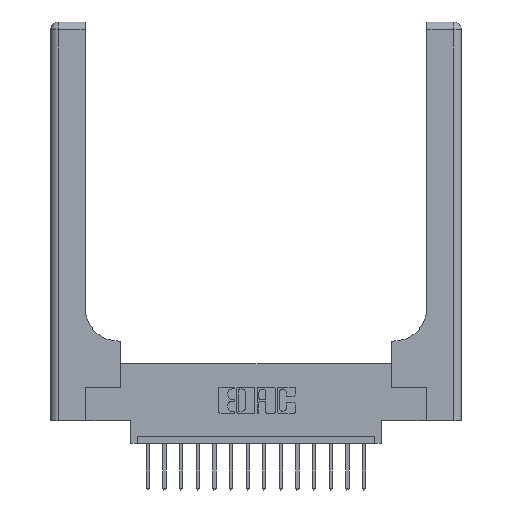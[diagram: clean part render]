
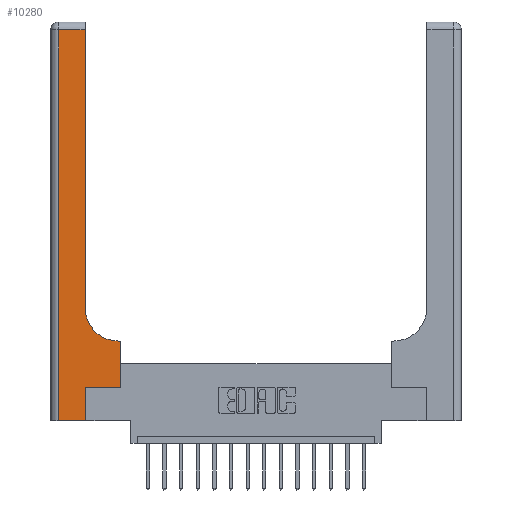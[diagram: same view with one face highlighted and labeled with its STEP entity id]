
A CAD part, top view. The second image highlights one B-rep face of the part: STEP entity #10280.
In plain terms, the highlighted planar face has unit normal (0, 0, 1).
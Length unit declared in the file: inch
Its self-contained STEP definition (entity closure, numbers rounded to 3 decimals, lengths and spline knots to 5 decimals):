
#17 = VERTEX_POINT ( 'NONE', #7320 ) ;
#414 = ORIENTED_EDGE ( 'NONE', *, *, #18149, .T. ) ;
#710 = VERTEX_POINT ( 'NONE', #17041 ) ;
#808 = EDGE_CURVE ( 'NONE', #9698, #7693, #7639, .T. ) ;
#989 = CARTESIAN_POINT ( 'NONE',  ( 0.06, 3., 0.37 ) ) ;
#1818 = ORIENTED_EDGE ( 'NONE', *, *, #17725, .T. ) ;
#1839 = CARTESIAN_POINT ( 'NONE',  ( 0., 3., 0.37 ) ) ;
#2275 = EDGE_CURVE ( 'NONE', #710, #17, #11465, .T. ) ;
#2359 = DIRECTION ( 'NONE',  ( 1., 0., 0. ) ) ;
#2383 = ORIENTED_EDGE ( 'NONE', *, *, #7016, .T. ) ;
#2452 = EDGE_CURVE ( 'NONE', #14809, #3536, #15968, .T. ) ;
#2605 = DIRECTION ( 'NONE',  ( 0., 0., -1. ) ) ;
#2976 = DIRECTION ( 'NONE',  ( 0., 1., 0. ) ) ;
#3241 = CARTESIAN_POINT ( 'NONE',  ( 0.265, 0., 0.37 ) ) ;
#3349 = DIRECTION ( 'NONE',  ( -1., 0., 0. ) ) ;
#3536 = VERTEX_POINT ( 'NONE', #13038 ) ;
#3635 = VERTEX_POINT ( 'NONE', #6782 ) ;
#3648 = CARTESIAN_POINT ( 'NONE',  ( 0.265, 0.25, 0.37 ) ) ;
#3989 = FACE_OUTER_BOUND ( 'NONE', #7374, .T. ) ;
#4073 = VERTEX_POINT ( 'NONE', #6824 ) ;
#4450 = ORIENTED_EDGE ( 'NONE', *, *, #2275, .T. ) ;
#4455 = ORIENTED_EDGE ( 'NONE', *, *, #808, .T. ) ;
#4923 = DIRECTION ( 'NONE',  ( -1., 0., 0. ) ) ;
#5470 = DIRECTION ( 'NONE',  ( -1., 0., 0. ) ) ;
#6045 = VECTOR ( 'NONE', #2976, 39.37008 ) ;
#6355 = CARTESIAN_POINT ( 'NONE',  ( 0.528, 0.25, 0.37 ) ) ;
#6574 = LINE ( 'NONE', #13385, #10532 ) ;
#6782 = CARTESIAN_POINT ( 'NONE',  ( 0.265, 0.25, 0.37 ) ) ;
#6824 = CARTESIAN_POINT ( 'NONE',  ( 0.528, 0.25, 0.37 ) ) ;
#7016 = EDGE_CURVE ( 'NONE', #3536, #710, #18098, .T. ) ;
#7320 = CARTESIAN_POINT ( 'NONE',  ( 0.26, 2.94, 0.37 ) ) ;
#7374 = EDGE_LOOP ( 'NONE', ( #4450, #15392, #4455, #16067, #1818, #414, #14215, #13484, #2383 ) ) ;
#7639 = LINE ( 'NONE', #989, #13537 ) ;
#7693 = VERTEX_POINT ( 'NONE', #14529 ) ;
#7717 = LINE ( 'NONE', #6355, #16822 ) ;
#7744 = EDGE_CURVE ( 'NONE', #4073, #14809, #7717, .T. ) ;
#8080 = CARTESIAN_POINT ( 'NONE',  ( 0.528, 0.6, 0.37 ) ) ;
#8204 = CARTESIAN_POINT ( 'NONE',  ( 0.265, 0., 0.37 ) ) ;
#8979 = CARTESIAN_POINT ( 'NONE',  ( 0.26, 0.6, 0.37 ) ) ;
#9279 = DIRECTION ( 'NONE',  ( 1., 0., 0. ) ) ;
#9527 = AXIS2_PLACEMENT_3D ( 'NONE', #1839, #2605, #5470 ) ;
#9698 = VERTEX_POINT ( 'NONE', #17572 ) ;
#9958 = VECTOR ( 'NONE', #13180, 39.37008 ) ;
#10175 = AXIS2_PLACEMENT_3D ( 'NONE', #11846, #11935, #9279 ) ;
#10280 = ADVANCED_FACE ( 'NONE', ( #3989 ), #12453, .F. ) ;
#10532 = VECTOR ( 'NONE', #4923, 39.37008 ) ;
#11465 = LINE ( 'NONE', #12646, #6045 ) ;
#11846 = CARTESIAN_POINT ( 'NONE',  ( 0.51, 0.85, 0.37 ) ) ;
#11883 = VERTEX_POINT ( 'NONE', #8204 ) ;
#11935 = DIRECTION ( 'NONE',  ( 0., 0., -1. ) ) ;
#12453 = PLANE ( 'NONE',  #9527 ) ;
#12646 = CARTESIAN_POINT ( 'NONE',  ( 0.26, 3., 0.37 ) ) ;
#13038 = CARTESIAN_POINT ( 'NONE',  ( 0.51, 0.6, 0.37 ) ) ;
#13091 = VECTOR ( 'NONE', #3349, 39.37008 ) ;
#13180 = DIRECTION ( 'NONE',  ( 0., 1., 0. ) ) ;
#13204 = VECTOR ( 'NONE', #2359, 39.37008 ) ;
#13230 = LINE ( 'NONE', #3648, #13204 ) ;
#13385 = CARTESIAN_POINT ( 'NONE',  ( 0., 2.94, 0.37 ) ) ;
#13432 = DIRECTION ( 'NONE',  ( 0., 1., 0. ) ) ;
#13484 = ORIENTED_EDGE ( 'NONE', *, *, #2452, .T. ) ;
#13537 = VECTOR ( 'NONE', #14901, 39.37008 ) ;
#14215 = ORIENTED_EDGE ( 'NONE', *, *, #7744, .T. ) ;
#14509 = DIRECTION ( 'NONE',  ( 1., 0., 0. ) ) ;
#14529 = CARTESIAN_POINT ( 'NONE',  ( 0.06, 0., 0.37 ) ) ;
#14809 = VERTEX_POINT ( 'NONE', #8080 ) ;
#14901 = DIRECTION ( 'NONE',  ( 0., -1., 0. ) ) ;
#15392 = ORIENTED_EDGE ( 'NONE', *, *, #16712, .T. ) ;
#15968 = LINE ( 'NONE', #8979, #13091 ) ;
#16067 = ORIENTED_EDGE ( 'NONE', *, *, #18022, .T. ) ;
#16712 = EDGE_CURVE ( 'NONE', #17, #9698, #6574, .T. ) ;
#16822 = VECTOR ( 'NONE', #13432, 39.37008 ) ;
#17041 = CARTESIAN_POINT ( 'NONE',  ( 0.26, 0.85, 0.37 ) ) ;
#17109 = LINE ( 'NONE', #17200, #17606 ) ;
#17200 = CARTESIAN_POINT ( 'NONE',  ( 0., 0., 0.37 ) ) ;
#17343 = LINE ( 'NONE', #3241, #9958 ) ;
#17572 = CARTESIAN_POINT ( 'NONE',  ( 0.06, 2.94, 0.37 ) ) ;
#17606 = VECTOR ( 'NONE', #14509, 39.37008 ) ;
#17725 = EDGE_CURVE ( 'NONE', #11883, #3635, #17343, .T. ) ;
#18022 = EDGE_CURVE ( 'NONE', #7693, #11883, #17109, .T. ) ;
#18098 = CIRCLE ( 'NONE', #10175, 0.25 ) ;
#18149 = EDGE_CURVE ( 'NONE', #3635, #4073, #13230, .T. ) ;
